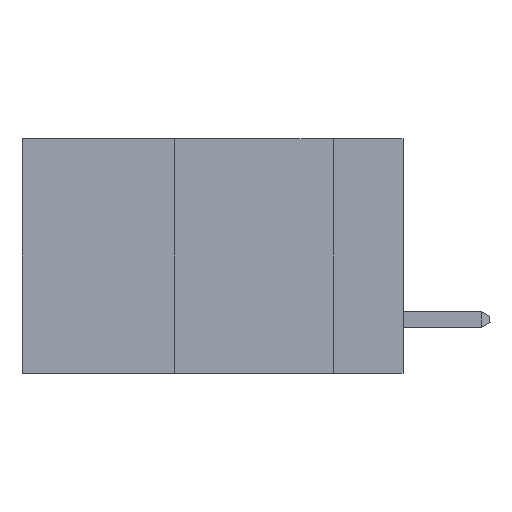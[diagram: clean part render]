
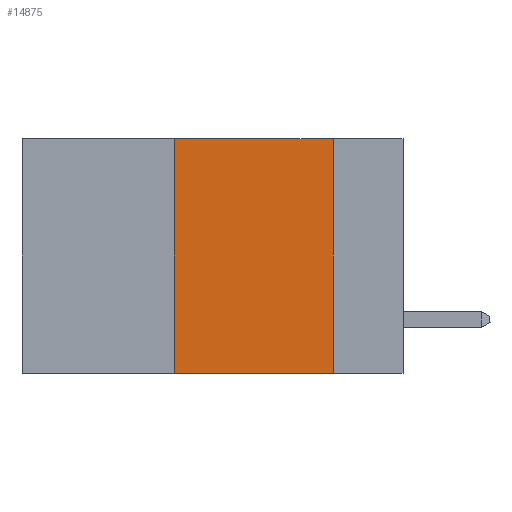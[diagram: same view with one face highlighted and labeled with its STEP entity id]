
A CAD part, left-side view. The second image highlights one B-rep face of the part: STEP entity #14875.
In plain terms, the highlighted planar face has unit normal (-1, 0, 0).
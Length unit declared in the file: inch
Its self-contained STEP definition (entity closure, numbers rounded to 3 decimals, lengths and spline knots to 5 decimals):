
#1352 = CARTESIAN_POINT ( 'NONE',  ( 0., 0.36, 0. ) ) ;
#1508 = LINE ( 'NONE', #7157, #41702 ) ;
#1849 = VERTEX_POINT ( 'NONE', #17223 ) ;
#3275 = DIRECTION ( 'NONE',  ( 1., 0., 0. ) ) ;
#3369 = EDGE_LOOP ( 'NONE', ( #46563, #48974, #32605, #8489 ) ) ;
#5772 = VERTEX_POINT ( 'NONE', #48339 ) ;
#7129 = VERTEX_POINT ( 'NONE', #33700 ) ;
#7157 = CARTESIAN_POINT ( 'NONE',  ( 0., 0.6, 0. ) ) ;
#8489 = ORIENTED_EDGE ( 'NONE', *, *, #30824, .T. ) ;
#14875 = ADVANCED_FACE ( 'NONE', ( #26740 ), #45913, .F. ) ;
#15530 = VERTEX_POINT ( 'NONE', #29242 ) ;
#16969 = AXIS2_PLACEMENT_3D ( 'NONE', #22889, #3275, #41693 ) ;
#17223 = CARTESIAN_POINT ( 'NONE',  ( 0., 0.36, 0. ) ) ;
#18196 = EDGE_CURVE ( 'NONE', #7129, #15530, #20262, .T. ) ;
#18339 = DIRECTION ( 'NONE',  ( 0., -1., 0. ) ) ;
#20262 = LINE ( 'NONE', #50010, #25163 ) ;
#20651 = LINE ( 'NONE', #1352, #33486 ) ;
#22889 = CARTESIAN_POINT ( 'NONE',  ( 0., 0.6, 0. ) ) ;
#25163 = VECTOR ( 'NONE', #46426, 39.37008 ) ;
#26550 = VECTOR ( 'NONE', #18339, 39.37008 ) ;
#26740 = FACE_OUTER_BOUND ( 'NONE', #3369, .T. ) ;
#28576 = DIRECTION ( 'NONE',  ( 0., 0., 1. ) ) ;
#29242 = CARTESIAN_POINT ( 'NONE',  ( 0., 0.11, -0.37 ) ) ;
#30824 = EDGE_CURVE ( 'NONE', #5772, #15530, #47112, .T. ) ;
#32605 = ORIENTED_EDGE ( 'NONE', *, *, #39983, .F. ) ;
#33053 = EDGE_CURVE ( 'NONE', #1849, #7129, #1508, .T. ) ;
#33486 = VECTOR ( 'NONE', #28576, 39.37008 ) ;
#33700 = CARTESIAN_POINT ( 'NONE',  ( 0., 0.11, 0. ) ) ;
#33924 = CARTESIAN_POINT ( 'NONE',  ( 0., 0.6, -0.37 ) ) ;
#39983 = EDGE_CURVE ( 'NONE', #5772, #1849, #20651, .T. ) ;
#41693 = DIRECTION ( 'NONE',  ( 0., 0., -1. ) ) ;
#41702 = VECTOR ( 'NONE', #47357, 39.37008 ) ;
#45913 = PLANE ( 'NONE',  #16969 ) ;
#46426 = DIRECTION ( 'NONE',  ( 0., 0., -1. ) ) ;
#46563 = ORIENTED_EDGE ( 'NONE', *, *, #18196, .F. ) ;
#47112 = LINE ( 'NONE', #33924, #26550 ) ;
#47357 = DIRECTION ( 'NONE',  ( 0., -1., 0. ) ) ;
#48339 = CARTESIAN_POINT ( 'NONE',  ( 0., 0.36, -0.37 ) ) ;
#48974 = ORIENTED_EDGE ( 'NONE', *, *, #33053, .F. ) ;
#50010 = CARTESIAN_POINT ( 'NONE',  ( 0., 0.11, 0. ) ) ;
